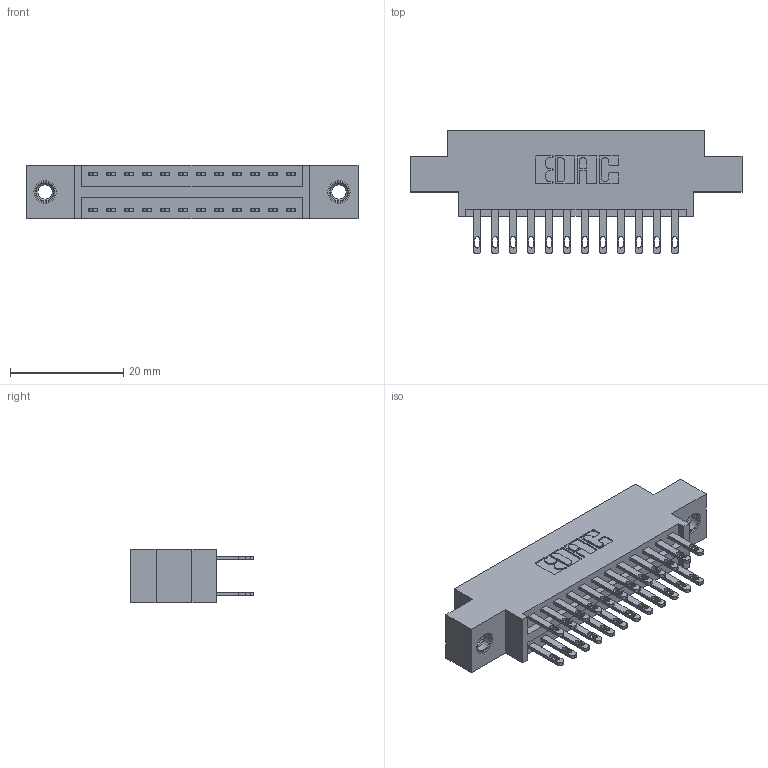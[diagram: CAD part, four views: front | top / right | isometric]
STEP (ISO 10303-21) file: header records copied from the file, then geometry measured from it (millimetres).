
FILE_DESCRIPTION (( 'STEP AP203' ), '1' );
FILE_NAME ('896-024-500-807.STEP', '2021-07-27T17:35:02', ( '' ), ( '' ), 'SwSTEP 2.0', 'SolidWorks 2020', '' );
FILE_SCHEMA (( 'CONFIG_CONTROL_DESIGN' ));
Length unit declared in the file: inch
Products named in the file (4): 846 Part_0.170 Offset - 0.156 Dia-TI; 896-024-500-807; 345-292-001_345-293-100; 345-250-001_345-250-005-103
Assembly tree (27 placements, depth 2):
  896-024-500-807
    846 Part_0.170 Offset - 0.156 Dia-TI
    345-292-001_345-293-100  x24
    345-250-001_345-250-005-103  x2
Bounding box: 58.67 x 21.84 x 9.4 mm (x, y, z)
Volume: 5393.7 mm3; surface area: 7407 mm2
Topology: 27 solids, 27 shells, 1338 faces, 4005 edges, 2662 vertices
Faces by surface type: plane 808, cylinder 514, cone 12, torus 4
Entity records: 13118 total; most frequent: CARTESIAN_POINT 2187, ORIENTED_EDGE 2114, DIRECTION 2007, EDGE_CURVE 1057, LINE 853, VECTOR 853, VERTEX_POINT 700, AXIS2_PLACEMENT_3D 577
